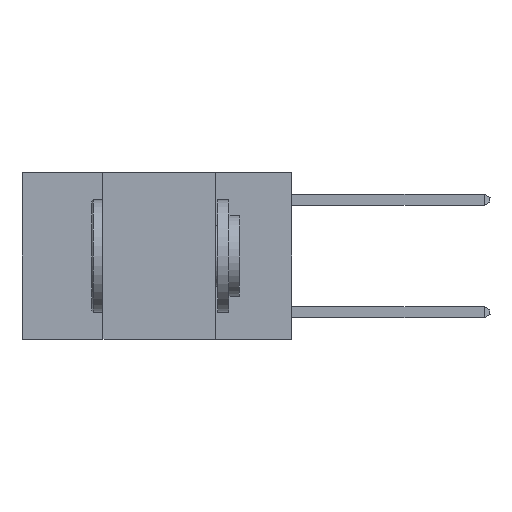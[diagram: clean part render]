
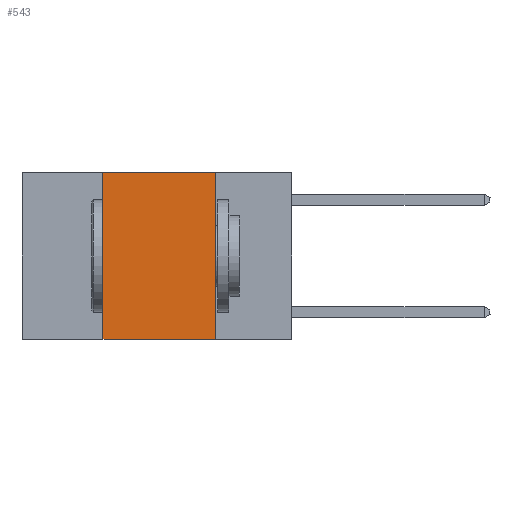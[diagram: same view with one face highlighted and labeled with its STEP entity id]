
A CAD part, left-side view. The second image highlights one B-rep face of the part: STEP entity #543.
In plain terms, the highlighted planar face has unit normal (-1, 0, 0).
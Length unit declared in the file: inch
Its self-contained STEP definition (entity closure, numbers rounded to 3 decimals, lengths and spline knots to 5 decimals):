
#91 = LINE ( 'NONE', #19776, #14599 ) ;
#543 = ADVANCED_FACE ( 'NONE', ( #13316 ), #13446, .F. ) ;
#1871 = ORIENTED_EDGE ( 'NONE', *, *, #18990, .F. ) ;
#2203 = ORIENTED_EDGE ( 'NONE', *, *, #2304, .F. ) ;
#2304 = EDGE_CURVE ( 'NONE', #18823, #16009, #4315, .T. ) ;
#2715 = VERTEX_POINT ( 'NONE', #18907 ) ;
#3308 = VERTEX_POINT ( 'NONE', #20134 ) ;
#3790 = DIRECTION ( 'NONE',  ( 0., 0., -1. ) ) ;
#3844 = VECTOR ( 'NONE', #7325, 39.37008 ) ;
#4315 = LINE ( 'NONE', #12370, #11284 ) ;
#5127 = EDGE_LOOP ( 'NONE', ( #1871, #2203, #16487, #7139 ) ) ;
#5745 = CARTESIAN_POINT ( 'NONE',  ( 0., 0.42, 0. ) ) ;
#5977 = VECTOR ( 'NONE', #7984, 39.37008 ) ;
#7139 = ORIENTED_EDGE ( 'NONE', *, *, #11769, .T. ) ;
#7325 = DIRECTION ( 'NONE',  ( 0., 0., -1. ) ) ;
#7984 = DIRECTION ( 'NONE',  ( 0., 0., 1. ) ) ;
#8807 = AXIS2_PLACEMENT_3D ( 'NONE', #15575, #23496, #3790 ) ;
#10367 = DIRECTION ( 'NONE',  ( 0., -1., 0. ) ) ;
#11284 = VECTOR ( 'NONE', #10367, 39.37008 ) ;
#11769 = EDGE_CURVE ( 'NONE', #2715, #3308, #91, .T. ) ;
#12370 = CARTESIAN_POINT ( 'NONE',  ( 0., 0.6, 0. ) ) ;
#13316 = FACE_OUTER_BOUND ( 'NONE', #5127, .T. ) ;
#13446 = PLANE ( 'NONE',  #8807 ) ;
#14599 = VECTOR ( 'NONE', #23988, 39.37008 ) ;
#15575 = CARTESIAN_POINT ( 'NONE',  ( 0., 0.6, 0. ) ) ;
#16009 = VERTEX_POINT ( 'NONE', #16058 ) ;
#16058 = CARTESIAN_POINT ( 'NONE',  ( 0., 0.17, 0. ) ) ;
#16487 = ORIENTED_EDGE ( 'NONE', *, *, #19969, .F. ) ;
#17755 = CARTESIAN_POINT ( 'NONE',  ( 0., 0.17, 0. ) ) ;
#18823 = VERTEX_POINT ( 'NONE', #21184 ) ;
#18907 = CARTESIAN_POINT ( 'NONE',  ( 0., 0.42, -0.37 ) ) ;
#18990 = EDGE_CURVE ( 'NONE', #16009, #3308, #23562, .T. ) ;
#19776 = CARTESIAN_POINT ( 'NONE',  ( 0., 0.6, -0.37 ) ) ;
#19969 = EDGE_CURVE ( 'NONE', #2715, #18823, #23859, .T. ) ;
#20134 = CARTESIAN_POINT ( 'NONE',  ( 0., 0.17, -0.37 ) ) ;
#21184 = CARTESIAN_POINT ( 'NONE',  ( 0., 0.42, 0. ) ) ;
#23496 = DIRECTION ( 'NONE',  ( 1., 0., 0. ) ) ;
#23562 = LINE ( 'NONE', #17755, #3844 ) ;
#23859 = LINE ( 'NONE', #5745, #5977 ) ;
#23988 = DIRECTION ( 'NONE',  ( 0., -1., 0. ) ) ;
